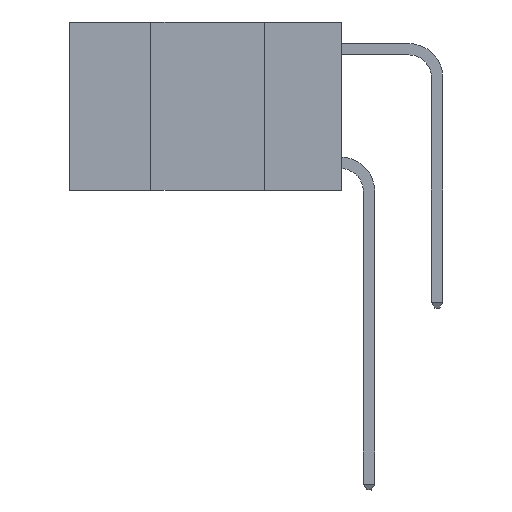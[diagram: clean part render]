
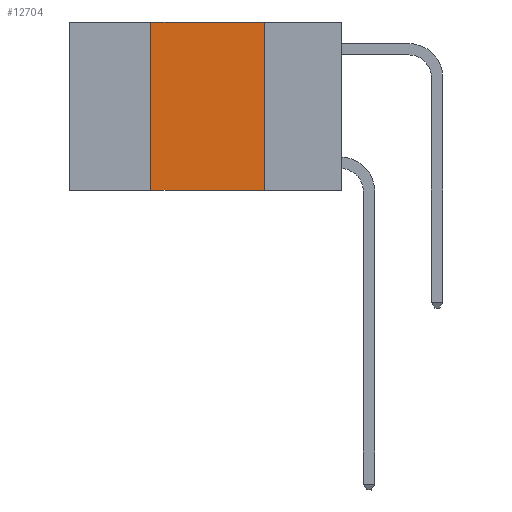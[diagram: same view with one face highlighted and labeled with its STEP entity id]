
A CAD part, left-side view. The second image highlights one B-rep face of the part: STEP entity #12704.
In plain terms, the highlighted planar face has unit normal (-1, 0, 0).
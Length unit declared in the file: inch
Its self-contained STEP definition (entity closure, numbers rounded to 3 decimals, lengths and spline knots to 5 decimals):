
#805 = ORIENTED_EDGE ( 'NONE', *, *, #4542, .F. ) ;
#975 = PLANE ( 'NONE',  #4551 ) ;
#1080 = ORIENTED_EDGE ( 'NONE', *, *, #1956, .F. ) ;
#1374 = LINE ( 'NONE', #1809, #13002 ) ;
#1809 = CARTESIAN_POINT ( 'NONE',  ( 0., 0.6, -0.37 ) ) ;
#1956 = EDGE_CURVE ( 'NONE', #3207, #3061, #10983, .T. ) ;
#2301 = EDGE_CURVE ( 'NONE', #3061, #9483, #3859, .T. ) ;
#2778 = EDGE_LOOP ( 'NONE', ( #6095, #1080, #805, #13686 ) ) ;
#3061 = VERTEX_POINT ( 'NONE', #8713 ) ;
#3207 = VERTEX_POINT ( 'NONE', #4984 ) ;
#3717 = DIRECTION ( 'NONE',  ( 0., 0., -1. ) ) ;
#3859 = LINE ( 'NONE', #14092, #11132 ) ;
#4542 = EDGE_CURVE ( 'NONE', #12160, #3207, #14190, .T. ) ;
#4551 = AXIS2_PLACEMENT_3D ( 'NONE', #6388, #5177, #3717 ) ;
#4984 = CARTESIAN_POINT ( 'NONE',  ( 0., 0.42, 0. ) ) ;
#5177 = DIRECTION ( 'NONE',  ( 1., 0., 0. ) ) ;
#5290 = DIRECTION ( 'NONE',  ( 0., -1., 0. ) ) ;
#6082 = CARTESIAN_POINT ( 'NONE',  ( 0., 0.42, -0.37 ) ) ;
#6095 = ORIENTED_EDGE ( 'NONE', *, *, #2301, .F. ) ;
#6158 = DIRECTION ( 'NONE',  ( 0., -1., 0. ) ) ;
#6388 = CARTESIAN_POINT ( 'NONE',  ( 0., 0.6, 0. ) ) ;
#6467 = DIRECTION ( 'NONE',  ( 0., 0., -1. ) ) ;
#7035 = DIRECTION ( 'NONE',  ( 0., 0., 1. ) ) ;
#7495 = EDGE_CURVE ( 'NONE', #12160, #9483, #1374, .T. ) ;
#8583 = CARTESIAN_POINT ( 'NONE',  ( 0., 0.17, -0.37 ) ) ;
#8713 = CARTESIAN_POINT ( 'NONE',  ( 0., 0.17, 0. ) ) ;
#9445 = CARTESIAN_POINT ( 'NONE',  ( 0., 0.6, 0. ) ) ;
#9483 = VERTEX_POINT ( 'NONE', #8583 ) ;
#10968 = VECTOR ( 'NONE', #6158, 39.37008 ) ;
#10983 = LINE ( 'NONE', #9445, #10968 ) ;
#11044 = VECTOR ( 'NONE', #7035, 39.37008 ) ;
#11132 = VECTOR ( 'NONE', #6467, 39.37008 ) ;
#11415 = CARTESIAN_POINT ( 'NONE',  ( 0., 0.42, 0. ) ) ;
#12160 = VERTEX_POINT ( 'NONE', #6082 ) ;
#12704 = ADVANCED_FACE ( 'NONE', ( #14309 ), #975, .F. ) ;
#13002 = VECTOR ( 'NONE', #5290, 39.37008 ) ;
#13686 = ORIENTED_EDGE ( 'NONE', *, *, #7495, .T. ) ;
#14092 = CARTESIAN_POINT ( 'NONE',  ( 0., 0.17, 0. ) ) ;
#14190 = LINE ( 'NONE', #11415, #11044 ) ;
#14309 = FACE_OUTER_BOUND ( 'NONE', #2778, .T. ) ;
